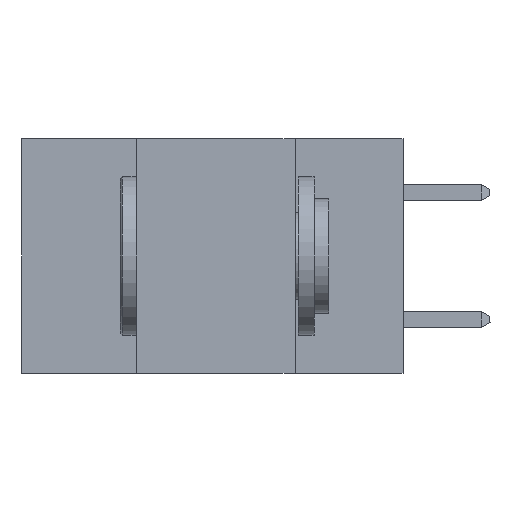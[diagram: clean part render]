
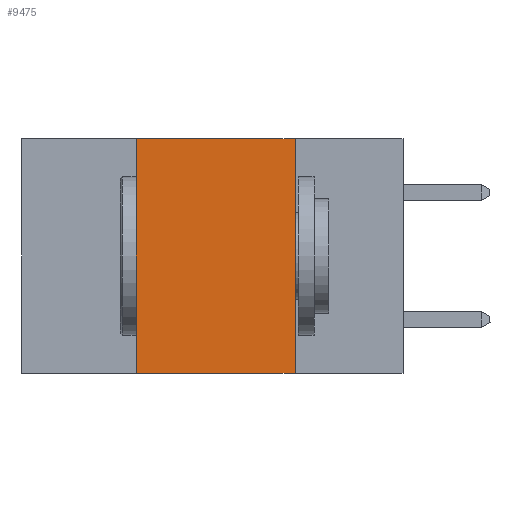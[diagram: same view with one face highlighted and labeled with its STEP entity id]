
A CAD part, left-side view. The second image highlights one B-rep face of the part: STEP entity #9475.
In plain terms, the highlighted planar face has unit normal (-1, 0, 0).
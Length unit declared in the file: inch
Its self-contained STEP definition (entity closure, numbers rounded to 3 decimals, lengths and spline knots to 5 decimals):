
#863 = EDGE_CURVE ( 'NONE', #4869, #4837, #14630, .T. ) ;
#1677 = EDGE_CURVE ( 'NONE', #10836, #4869, #3956, .T. ) ;
#1779 = CARTESIAN_POINT ( 'NONE',  ( 0., 0.42, -0.37 ) ) ;
#1887 = DIRECTION ( 'NONE',  ( 0., 0., -1. ) ) ;
#1936 = DIRECTION ( 'NONE',  ( 1., 0., 0. ) ) ;
#2529 = AXIS2_PLACEMENT_3D ( 'NONE', #5217, #1936, #1887 ) ;
#2615 = EDGE_CURVE ( 'NONE', #5796, #10836, #4672, .T. ) ;
#2964 = DIRECTION ( 'NONE',  ( 0., 0., 1. ) ) ;
#3196 = CARTESIAN_POINT ( 'NONE',  ( 0., 0.17, -0.37 ) ) ;
#3956 = LINE ( 'NONE', #6963, #6819 ) ;
#3966 = EDGE_CURVE ( 'NONE', #5796, #4837, #7892, .T. ) ;
#4672 = LINE ( 'NONE', #10563, #12025 ) ;
#4837 = VERTEX_POINT ( 'NONE', #3196 ) ;
#4869 = VERTEX_POINT ( 'NONE', #11505 ) ;
#5217 = CARTESIAN_POINT ( 'NONE',  ( 0., 0.6, 0. ) ) ;
#5781 = EDGE_LOOP ( 'NONE', ( #9232, #9858, #13541, #13381 ) ) ;
#5796 = VERTEX_POINT ( 'NONE', #1779 ) ;
#6819 = VECTOR ( 'NONE', #8124, 39.37008 ) ;
#6963 = CARTESIAN_POINT ( 'NONE',  ( 0., 0.6, 0. ) ) ;
#7892 = LINE ( 'NONE', #9570, #9325 ) ;
#8124 = DIRECTION ( 'NONE',  ( 0., -1., 0. ) ) ;
#9232 = ORIENTED_EDGE ( 'NONE', *, *, #863, .F. ) ;
#9325 = VECTOR ( 'NONE', #14281, 39.37008 ) ;
#9368 = VECTOR ( 'NONE', #12514, 39.37008 ) ;
#9475 = ADVANCED_FACE ( 'NONE', ( #12975 ), #10952, .F. ) ;
#9570 = CARTESIAN_POINT ( 'NONE',  ( 0., 0.6, -0.37 ) ) ;
#9858 = ORIENTED_EDGE ( 'NONE', *, *, #1677, .F. ) ;
#10563 = CARTESIAN_POINT ( 'NONE',  ( 0., 0.42, 0. ) ) ;
#10836 = VERTEX_POINT ( 'NONE', #11145 ) ;
#10952 = PLANE ( 'NONE',  #2529 ) ;
#11145 = CARTESIAN_POINT ( 'NONE',  ( 0., 0.42, 0. ) ) ;
#11505 = CARTESIAN_POINT ( 'NONE',  ( 0., 0.17, 0. ) ) ;
#12025 = VECTOR ( 'NONE', #2964, 39.37008 ) ;
#12514 = DIRECTION ( 'NONE',  ( 0., 0., -1. ) ) ;
#12975 = FACE_OUTER_BOUND ( 'NONE', #5781, .T. ) ;
#13308 = CARTESIAN_POINT ( 'NONE',  ( 0., 0.17, 0. ) ) ;
#13381 = ORIENTED_EDGE ( 'NONE', *, *, #3966, .T. ) ;
#13541 = ORIENTED_EDGE ( 'NONE', *, *, #2615, .F. ) ;
#14281 = DIRECTION ( 'NONE',  ( 0., -1., 0. ) ) ;
#14630 = LINE ( 'NONE', #13308, #9368 ) ;
